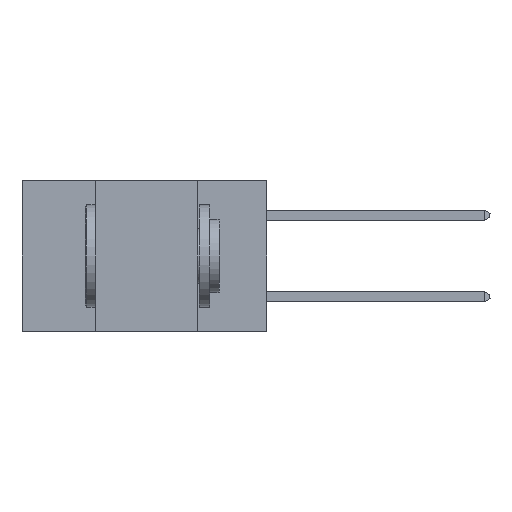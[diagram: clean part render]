
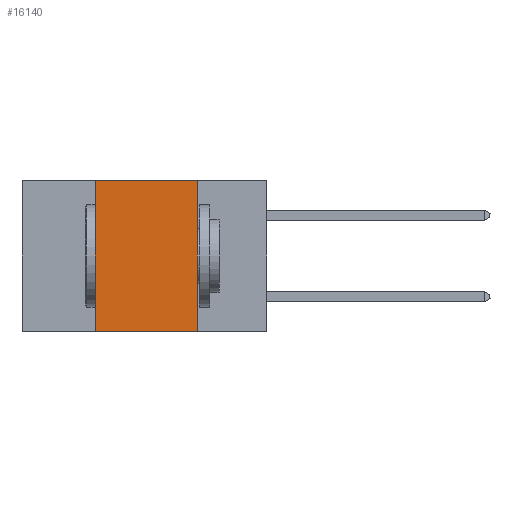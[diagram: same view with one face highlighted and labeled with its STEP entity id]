
A CAD part, left-side view. The second image highlights one B-rep face of the part: STEP entity #16140.
In plain terms, the highlighted planar face has unit normal (-1, 0, 0).
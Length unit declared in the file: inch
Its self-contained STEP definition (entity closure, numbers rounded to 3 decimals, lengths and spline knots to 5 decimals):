
#518 = EDGE_CURVE ( 'NONE', #14057, #3160, #15817, .T. ) ;
#598 = CARTESIAN_POINT ( 'NONE',  ( 0., 0.6, 0. ) ) ;
#958 = EDGE_CURVE ( 'NONE', #3160, #8341, #13628, .T. ) ;
#1987 = ORIENTED_EDGE ( 'NONE', *, *, #11742, .T. ) ;
#2024 = DIRECTION ( 'NONE',  ( 0., -1., 0. ) ) ;
#3160 = VERTEX_POINT ( 'NONE', #5601 ) ;
#3292 = VECTOR ( 'NONE', #2024, 39.37008 ) ;
#3963 = FACE_OUTER_BOUND ( 'NONE', #14395, .T. ) ;
#4727 = CARTESIAN_POINT ( 'NONE',  ( 0., 0.17, -0.37 ) ) ;
#5601 = CARTESIAN_POINT ( 'NONE',  ( 0., 0.42, 0. ) ) ;
#6828 = PLANE ( 'NONE',  #6914 ) ;
#6914 = AXIS2_PLACEMENT_3D ( 'NONE', #14601, #15875, #8129 ) ;
#6993 = EDGE_CURVE ( 'NONE', #8341, #12767, #8586, .T. ) ;
#7064 = CARTESIAN_POINT ( 'NONE',  ( 0., 0.42, -0.37 ) ) ;
#7715 = CARTESIAN_POINT ( 'NONE',  ( 0., 0.17, 0. ) ) ;
#8071 = ORIENTED_EDGE ( 'NONE', *, *, #6993, .F. ) ;
#8129 = DIRECTION ( 'NONE',  ( 0., 0., -1. ) ) ;
#8176 = VECTOR ( 'NONE', #12218, 39.37008 ) ;
#8341 = VERTEX_POINT ( 'NONE', #7715 ) ;
#8586 = LINE ( 'NONE', #10881, #8176 ) ;
#9595 = VECTOR ( 'NONE', #16862, 39.37008 ) ;
#10236 = CARTESIAN_POINT ( 'NONE',  ( 0., 0.42, 0. ) ) ;
#10517 = DIRECTION ( 'NONE',  ( 0., 0., 1. ) ) ;
#10881 = CARTESIAN_POINT ( 'NONE',  ( 0., 0.17, 0. ) ) ;
#11742 = EDGE_CURVE ( 'NONE', #14057, #12767, #16435, .T. ) ;
#11798 = CARTESIAN_POINT ( 'NONE',  ( 0., 0.6, -0.37 ) ) ;
#11985 = VECTOR ( 'NONE', #10517, 39.37008 ) ;
#12218 = DIRECTION ( 'NONE',  ( 0., 0., -1. ) ) ;
#12767 = VERTEX_POINT ( 'NONE', #4727 ) ;
#13628 = LINE ( 'NONE', #598, #3292 ) ;
#14057 = VERTEX_POINT ( 'NONE', #7064 ) ;
#14395 = EDGE_LOOP ( 'NONE', ( #8071, #14967, #15367, #1987 ) ) ;
#14601 = CARTESIAN_POINT ( 'NONE',  ( 0., 0.6, 0. ) ) ;
#14967 = ORIENTED_EDGE ( 'NONE', *, *, #958, .F. ) ;
#15367 = ORIENTED_EDGE ( 'NONE', *, *, #518, .F. ) ;
#15817 = LINE ( 'NONE', #10236, #11985 ) ;
#15875 = DIRECTION ( 'NONE',  ( 1., 0., 0. ) ) ;
#16140 = ADVANCED_FACE ( 'NONE', ( #3963 ), #6828, .F. ) ;
#16435 = LINE ( 'NONE', #11798, #9595 ) ;
#16862 = DIRECTION ( 'NONE',  ( 0., -1., 0. ) ) ;
